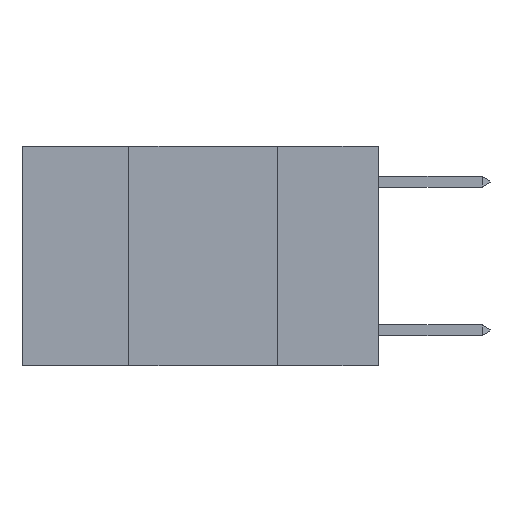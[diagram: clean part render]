
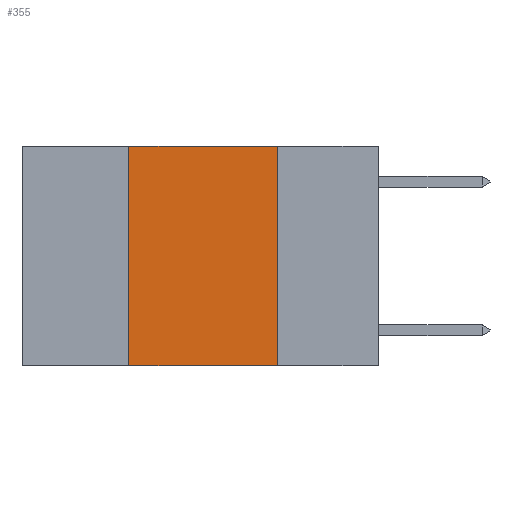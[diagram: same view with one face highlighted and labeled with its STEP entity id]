
A CAD part, left-side view. The second image highlights one B-rep face of the part: STEP entity #355.
In plain terms, the highlighted planar face has unit normal (-1, 0, 0).
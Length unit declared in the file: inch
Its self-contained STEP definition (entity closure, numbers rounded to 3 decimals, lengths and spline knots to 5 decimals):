
#203 = CARTESIAN_POINT ( 'NONE',  ( 0., 0.17, -0.37 ) ) ;
#355 = ADVANCED_FACE ( 'NONE', ( #3734 ), #12496, .F. ) ;
#516 = DIRECTION ( 'NONE',  ( 0., 0., -1. ) ) ;
#942 = LINE ( 'NONE', #5345, #5884 ) ;
#952 = CARTESIAN_POINT ( 'NONE',  ( 0., 0.42, 0. ) ) ;
#1629 = DIRECTION ( 'NONE',  ( 0., -1., 0. ) ) ;
#2416 = EDGE_CURVE ( 'NONE', #3337, #10513, #8067, .T. ) ;
#2614 = VERTEX_POINT ( 'NONE', #10894 ) ;
#2651 = CARTESIAN_POINT ( 'NONE',  ( 0., 0.6, 0. ) ) ;
#3333 = DIRECTION ( 'NONE',  ( 0., -1., 0. ) ) ;
#3337 = VERTEX_POINT ( 'NONE', #12783 ) ;
#3532 = ORIENTED_EDGE ( 'NONE', *, *, #11939, .F. ) ;
#3734 = FACE_OUTER_BOUND ( 'NONE', #8525, .T. ) ;
#4052 = LINE ( 'NONE', #8414, #8146 ) ;
#4507 = ORIENTED_EDGE ( 'NONE', *, *, #2416, .T. ) ;
#5231 = LINE ( 'NONE', #952, #12847 ) ;
#5299 = DIRECTION ( 'NONE',  ( 0., 0., 1. ) ) ;
#5345 = CARTESIAN_POINT ( 'NONE',  ( 0., 0.6, 0. ) ) ;
#5884 = VECTOR ( 'NONE', #3333, 39.37008 ) ;
#6021 = ORIENTED_EDGE ( 'NONE', *, *, #11638, .F. ) ;
#6343 = AXIS2_PLACEMENT_3D ( 'NONE', #2651, #13568, #516 ) ;
#7490 = EDGE_CURVE ( 'NONE', #3337, #12148, #5231, .T. ) ;
#7833 = ORIENTED_EDGE ( 'NONE', *, *, #7490, .F. ) ;
#8067 = LINE ( 'NONE', #11402, #13189 ) ;
#8146 = VECTOR ( 'NONE', #12751, 39.37008 ) ;
#8414 = CARTESIAN_POINT ( 'NONE',  ( 0., 0.17, 0. ) ) ;
#8525 = EDGE_LOOP ( 'NONE', ( #3532, #6021, #7833, #4507 ) ) ;
#9941 = CARTESIAN_POINT ( 'NONE',  ( 0., 0.42, 0. ) ) ;
#10513 = VERTEX_POINT ( 'NONE', #203 ) ;
#10894 = CARTESIAN_POINT ( 'NONE',  ( 0., 0.17, 0. ) ) ;
#11402 = CARTESIAN_POINT ( 'NONE',  ( 0., 0.6, -0.37 ) ) ;
#11638 = EDGE_CURVE ( 'NONE', #12148, #2614, #942, .T. ) ;
#11939 = EDGE_CURVE ( 'NONE', #2614, #10513, #4052, .T. ) ;
#12148 = VERTEX_POINT ( 'NONE', #9941 ) ;
#12496 = PLANE ( 'NONE',  #6343 ) ;
#12751 = DIRECTION ( 'NONE',  ( 0., 0., -1. ) ) ;
#12783 = CARTESIAN_POINT ( 'NONE',  ( 0., 0.42, -0.37 ) ) ;
#12847 = VECTOR ( 'NONE', #5299, 39.37008 ) ;
#13189 = VECTOR ( 'NONE', #1629, 39.37008 ) ;
#13568 = DIRECTION ( 'NONE',  ( 1., 0., 0. ) ) ;
